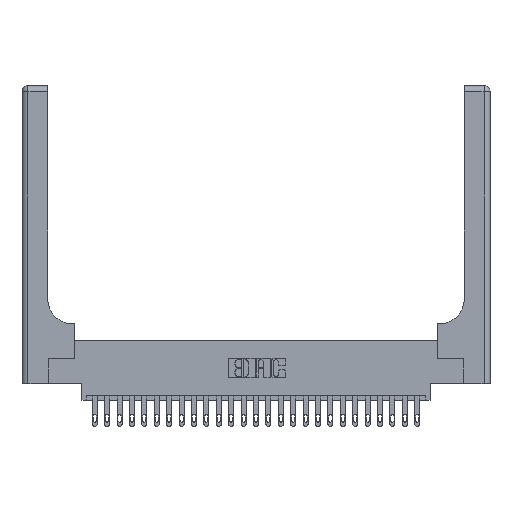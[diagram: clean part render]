
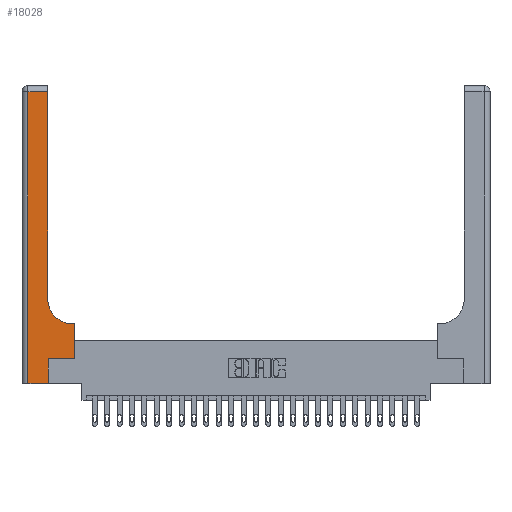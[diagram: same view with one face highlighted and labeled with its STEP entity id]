
A CAD part, top view. The second image highlights one B-rep face of the part: STEP entity #18028.
In plain terms, the highlighted planar face has unit normal (0, 0, 1).
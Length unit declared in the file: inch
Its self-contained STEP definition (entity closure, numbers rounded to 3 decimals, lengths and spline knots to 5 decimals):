
#389 = PLANE ( 'NONE',  #19872 ) ;
#564 = EDGE_CURVE ( 'NONE', #24656, #22735, #8189, .T. ) ;
#946 = LINE ( 'NONE', #24445, #22970 ) ;
#1015 = VERTEX_POINT ( 'NONE', #21002 ) ;
#1229 = CARTESIAN_POINT ( 'NONE',  ( 0.06, 2.94, 0.37 ) ) ;
#2158 = CARTESIAN_POINT ( 'NONE',  ( 0., 3., 0.37 ) ) ;
#2638 = VERTEX_POINT ( 'NONE', #5305 ) ;
#3234 = ORIENTED_EDGE ( 'NONE', *, *, #19311, .T. ) ;
#3358 = CARTESIAN_POINT ( 'NONE',  ( 0., 0., 0.37 ) ) ;
#3476 = CARTESIAN_POINT ( 'NONE',  ( 0.528, 0.6, 0.37 ) ) ;
#3848 = CARTESIAN_POINT ( 'NONE',  ( 0.265, 0., 0.37 ) ) ;
#4212 = EDGE_CURVE ( 'NONE', #6060, #25313, #20325, .T. ) ;
#4358 = EDGE_CURVE ( 'NONE', #25313, #13743, #24568, .T. ) ;
#5273 = DIRECTION ( 'NONE',  ( 0., 1., 0. ) ) ;
#5305 = CARTESIAN_POINT ( 'NONE',  ( 0.26, 2.94, 0.37 ) ) ;
#5818 = VECTOR ( 'NONE', #5273, 39.37008 ) ;
#5920 = ORIENTED_EDGE ( 'NONE', *, *, #23908, .T. ) ;
#6060 = VERTEX_POINT ( 'NONE', #1229 ) ;
#6548 = EDGE_CURVE ( 'NONE', #2638, #6060, #22988, .T. ) ;
#6622 = CARTESIAN_POINT ( 'NONE',  ( 0.265, 0.25, 0.37 ) ) ;
#6629 = EDGE_CURVE ( 'NONE', #8614, #1015, #15382, .T. ) ;
#6848 = DIRECTION ( 'NONE',  ( 0., 1., 0. ) ) ;
#7664 = DIRECTION ( 'NONE',  ( 1., 0., 0. ) ) ;
#7813 = FACE_OUTER_BOUND ( 'NONE', #23904, .T. ) ;
#7896 = AXIS2_PLACEMENT_3D ( 'NONE', #11121, #21392, #7664 ) ;
#8189 = LINE ( 'NONE', #17930, #23950 ) ;
#8417 = ORIENTED_EDGE ( 'NONE', *, *, #6629, .T. ) ;
#8614 = VERTEX_POINT ( 'NONE', #6622 ) ;
#9035 = ORIENTED_EDGE ( 'NONE', *, *, #564, .T. ) ;
#9085 = ORIENTED_EDGE ( 'NONE', *, *, #24691, .T. ) ;
#9122 = EDGE_CURVE ( 'NONE', #19083, #2638, #946, .T. ) ;
#9577 = CARTESIAN_POINT ( 'NONE',  ( 0.51, 0.6, 0.37 ) ) ;
#10158 = ORIENTED_EDGE ( 'NONE', *, *, #4212, .T. ) ;
#10196 = CARTESIAN_POINT ( 'NONE',  ( 0.265, 0., 0.37 ) ) ;
#10788 = DIRECTION ( 'NONE',  ( -1., 0., 0. ) ) ;
#11121 = CARTESIAN_POINT ( 'NONE',  ( 0.51, 0.85, 0.37 ) ) ;
#11901 = CARTESIAN_POINT ( 'NONE',  ( 0.265, 0.25, 0.37 ) ) ;
#12055 = VECTOR ( 'NONE', #12734, 39.37008 ) ;
#12059 = VECTOR ( 'NONE', #21181, 39.37008 ) ;
#12734 = DIRECTION ( 'NONE',  ( 0., -1., 0. ) ) ;
#12964 = VECTOR ( 'NONE', #21085, 39.37008 ) ;
#13443 = ORIENTED_EDGE ( 'NONE', *, *, #6548, .T. ) ;
#13705 = DIRECTION ( 'NONE',  ( -1., 0., 0. ) ) ;
#13743 = VERTEX_POINT ( 'NONE', #10196 ) ;
#14012 = CARTESIAN_POINT ( 'NONE',  ( 0.26, 0.85, 0.37 ) ) ;
#15129 = ORIENTED_EDGE ( 'NONE', *, *, #9122, .T. ) ;
#15154 = DIRECTION ( 'NONE',  ( 1., 0., 0. ) ) ;
#15382 = LINE ( 'NONE', #11901, #12059 ) ;
#15605 = DIRECTION ( 'NONE',  ( -1., 0., 0. ) ) ;
#15659 = CIRCLE ( 'NONE', #7896, 0.25 ) ;
#17930 = CARTESIAN_POINT ( 'NONE',  ( 0.26, 0.6, 0.37 ) ) ;
#18028 = ADVANCED_FACE ( 'NONE', ( #7813 ), #389, .F. ) ;
#19083 = VERTEX_POINT ( 'NONE', #14012 ) ;
#19311 = EDGE_CURVE ( 'NONE', #1015, #24656, #22766, .T. ) ;
#19850 = VECTOR ( 'NONE', #15154, 39.37008 ) ;
#19868 = DIRECTION ( 'NONE',  ( 0., 0., -1. ) ) ;
#19872 = AXIS2_PLACEMENT_3D ( 'NONE', #2158, #19868, #13705 ) ;
#19897 = VECTOR ( 'NONE', #10788, 39.37008 ) ;
#20325 = LINE ( 'NONE', #24448, #12055 ) ;
#20533 = CARTESIAN_POINT ( 'NONE',  ( 0., 2.94, 0.37 ) ) ;
#21002 = CARTESIAN_POINT ( 'NONE',  ( 0.528, 0.25, 0.37 ) ) ;
#21085 = DIRECTION ( 'NONE',  ( 0., 1., 0. ) ) ;
#21181 = DIRECTION ( 'NONE',  ( 1., 0., 0. ) ) ;
#21392 = DIRECTION ( 'NONE',  ( 0., 0., -1. ) ) ;
#21441 = LINE ( 'NONE', #3848, #5818 ) ;
#22735 = VERTEX_POINT ( 'NONE', #9577 ) ;
#22766 = LINE ( 'NONE', #23021, #12964 ) ;
#22970 = VECTOR ( 'NONE', #6848, 39.37008 ) ;
#22988 = LINE ( 'NONE', #20533, #19897 ) ;
#23019 = ORIENTED_EDGE ( 'NONE', *, *, #4358, .T. ) ;
#23021 = CARTESIAN_POINT ( 'NONE',  ( 0.528, 0.25, 0.37 ) ) ;
#23904 = EDGE_LOOP ( 'NONE', ( #15129, #13443, #10158, #23019, #9085, #8417, #3234, #9035, #5920 ) ) ;
#23908 = EDGE_CURVE ( 'NONE', #22735, #19083, #15659, .T. ) ;
#23950 = VECTOR ( 'NONE', #15605, 39.37008 ) ;
#24445 = CARTESIAN_POINT ( 'NONE',  ( 0.26, 3., 0.37 ) ) ;
#24448 = CARTESIAN_POINT ( 'NONE',  ( 0.06, 3., 0.37 ) ) ;
#24568 = LINE ( 'NONE', #3358, #19850 ) ;
#24656 = VERTEX_POINT ( 'NONE', #3476 ) ;
#24691 = EDGE_CURVE ( 'NONE', #13743, #8614, #21441, .T. ) ;
#25171 = CARTESIAN_POINT ( 'NONE',  ( 0.06, 0., 0.37 ) ) ;
#25313 = VERTEX_POINT ( 'NONE', #25171 ) ;
